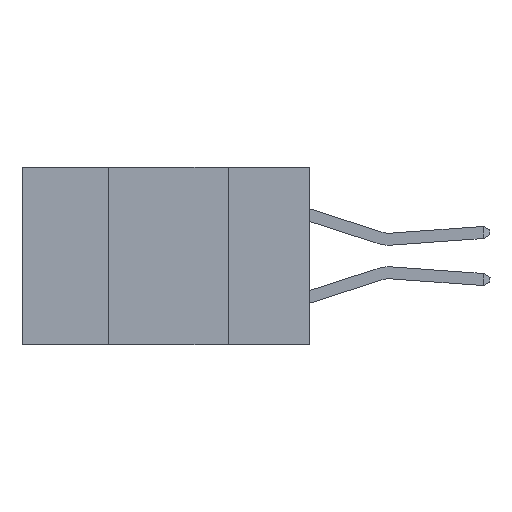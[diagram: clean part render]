
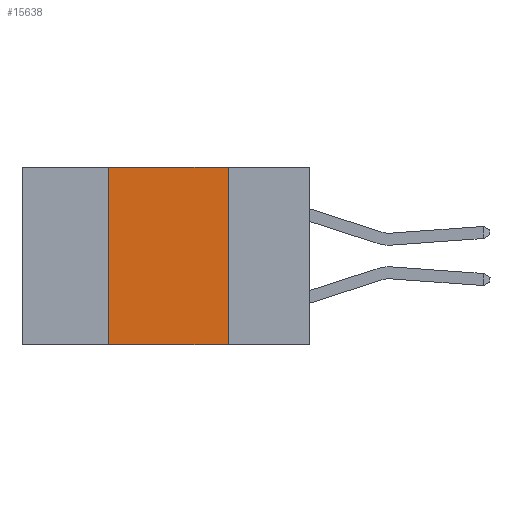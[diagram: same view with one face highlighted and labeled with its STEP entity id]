
A CAD part, left-side view. The second image highlights one B-rep face of the part: STEP entity #15638.
In plain terms, the highlighted planar face has unit normal (-1, 0, 0).
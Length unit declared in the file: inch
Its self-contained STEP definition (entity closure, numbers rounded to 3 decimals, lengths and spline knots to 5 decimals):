
#444 = DIRECTION ( 'NONE',  ( 0., 0., -1. ) ) ;
#485 = EDGE_CURVE ( 'NONE', #6298, #11595, #6228, .T. ) ;
#850 = AXIS2_PLACEMENT_3D ( 'NONE', #964, #12501, #3926 ) ;
#964 = CARTESIAN_POINT ( 'NONE',  ( 0., 0.6, 0. ) ) ;
#1106 = ORIENTED_EDGE ( 'NONE', *, *, #5025, .T. ) ;
#1458 = VECTOR ( 'NONE', #4137, 39.37008 ) ;
#1820 = CARTESIAN_POINT ( 'NONE',  ( 0., 0.6, -0.37 ) ) ;
#2269 = CARTESIAN_POINT ( 'NONE',  ( 0., 0.42, 0. ) ) ;
#2682 = ORIENTED_EDGE ( 'NONE', *, *, #14618, .F. ) ;
#2873 = VERTEX_POINT ( 'NONE', #2269 ) ;
#3253 = VECTOR ( 'NONE', #12975, 39.37008 ) ;
#3351 = EDGE_LOOP ( 'NONE', ( #4077, #2682, #18224, #1106 ) ) ;
#3926 = DIRECTION ( 'NONE',  ( 0., 0., -1. ) ) ;
#4077 = ORIENTED_EDGE ( 'NONE', *, *, #485, .F. ) ;
#4137 = DIRECTION ( 'NONE',  ( 0., -1., 0. ) ) ;
#5025 = EDGE_CURVE ( 'NONE', #5642, #11595, #12923, .T. ) ;
#5642 = VERTEX_POINT ( 'NONE', #18418 ) ;
#6228 = LINE ( 'NONE', #16402, #18400 ) ;
#6298 = VERTEX_POINT ( 'NONE', #14959 ) ;
#7081 = LINE ( 'NONE', #10143, #3253 ) ;
#7576 = EDGE_CURVE ( 'NONE', #5642, #2873, #11281, .T. ) ;
#8248 = DIRECTION ( 'NONE',  ( 0., 0., 1. ) ) ;
#8299 = CARTESIAN_POINT ( 'NONE',  ( 0., 0.42, -0.37 ) ) ;
#10143 = CARTESIAN_POINT ( 'NONE',  ( 0., 0.6, 0. ) ) ;
#11281 = LINE ( 'NONE', #8299, #18269 ) ;
#11595 = VERTEX_POINT ( 'NONE', #18003 ) ;
#12191 = FACE_OUTER_BOUND ( 'NONE', #3351, .T. ) ;
#12501 = DIRECTION ( 'NONE',  ( 1., 0., 0. ) ) ;
#12923 = LINE ( 'NONE', #1820, #1458 ) ;
#12975 = DIRECTION ( 'NONE',  ( 0., -1., 0. ) ) ;
#14618 = EDGE_CURVE ( 'NONE', #2873, #6298, #7081, .T. ) ;
#14959 = CARTESIAN_POINT ( 'NONE',  ( 0., 0.17, 0. ) ) ;
#15638 = ADVANCED_FACE ( 'NONE', ( #12191 ), #18054, .F. ) ;
#16402 = CARTESIAN_POINT ( 'NONE',  ( 0., 0.17, -0.37 ) ) ;
#18003 = CARTESIAN_POINT ( 'NONE',  ( 0., 0.17, -0.37 ) ) ;
#18054 = PLANE ( 'NONE',  #850 ) ;
#18224 = ORIENTED_EDGE ( 'NONE', *, *, #7576, .F. ) ;
#18269 = VECTOR ( 'NONE', #8248, 39.37008 ) ;
#18400 = VECTOR ( 'NONE', #444, 39.37008 ) ;
#18418 = CARTESIAN_POINT ( 'NONE',  ( 0., 0.42, -0.37 ) ) ;
